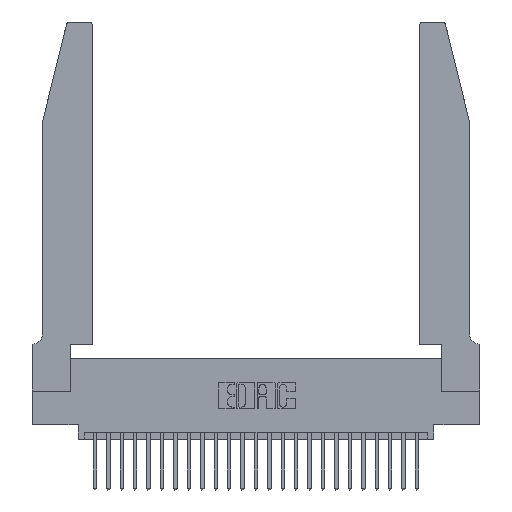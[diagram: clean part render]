
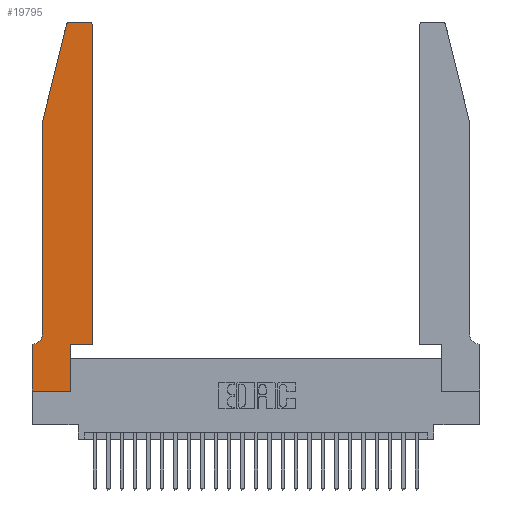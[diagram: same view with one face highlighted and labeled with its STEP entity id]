
A CAD part, top view. The second image highlights one B-rep face of the part: STEP entity #19795.
In plain terms, the highlighted planar face has unit normal (0, 0, 1).
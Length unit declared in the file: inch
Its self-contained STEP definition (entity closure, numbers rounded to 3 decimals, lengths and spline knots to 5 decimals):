
#88 = ORIENTED_EDGE ( 'NONE', *, *, #620, .T. ) ;
#238 = DIRECTION ( 'NONE',  ( 1., 0., 0. ) ) ;
#620 = EDGE_CURVE ( 'NONE', #8522, #22157, #18849, .T. ) ;
#905 = AXIS2_PLACEMENT_3D ( 'NONE', #3221, #17809, #5351 ) ;
#1166 = VECTOR ( 'NONE', #2863, 39.37008 ) ;
#1327 = VERTEX_POINT ( 'NONE', #24471 ) ;
#1481 = EDGE_CURVE ( 'NONE', #4591, #10371, #6172, .T. ) ;
#1505 = DIRECTION ( 'NONE',  ( 0., 1., 0. ) ) ;
#1758 = CARTESIAN_POINT ( 'NONE',  ( 0.0755, 0.35, 0.37 ) ) ;
#1765 = CARTESIAN_POINT ( 'NONE',  ( 0.2865, 0., 0.37 ) ) ;
#1898 = VECTOR ( 'NONE', #26459, 39.37008 ) ;
#2162 = ORIENTED_EDGE ( 'NONE', *, *, #11137, .T. ) ;
#2335 = VERTEX_POINT ( 'NONE', #6786 ) ;
#2593 = PLANE ( 'NONE',  #16353 ) ;
#2817 = LINE ( 'NONE', #15423, #1166 ) ;
#2863 = DIRECTION ( 'NONE',  ( 0., 1., 0. ) ) ;
#3044 = EDGE_CURVE ( 'NONE', #8219, #8522, #7078, .T. ) ;
#3221 = CARTESIAN_POINT ( 'NONE',  ( 0.4205, 2.72, 0.37 ) ) ;
#3338 = DIRECTION ( 'NONE',  ( 0., -1., 0. ) ) ;
#3476 = DIRECTION ( 'NONE',  ( 0., 0., -1. ) ) ;
#3484 = VECTOR ( 'NONE', #13917, 39.37008 ) ;
#4347 = ORIENTED_EDGE ( 'NONE', *, *, #3044, .T. ) ;
#4591 = VERTEX_POINT ( 'NONE', #17254 ) ;
#5323 = VECTOR ( 'NONE', #1505, 39.37008 ) ;
#5351 = DIRECTION ( 'NONE',  ( 1., 0., 0. ) ) ;
#6013 = LINE ( 'NONE', #14112, #5323 ) ;
#6172 = LINE ( 'NONE', #14824, #10483 ) ;
#6718 = CARTESIAN_POINT ( 'NONE',  ( 0.284, 2.72, 0.37 ) ) ;
#6786 = CARTESIAN_POINT ( 'NONE',  ( 0.4505, 2.72, 0.37 ) ) ;
#7078 = LINE ( 'NONE', #23524, #12006 ) ;
#7126 = ORIENTED_EDGE ( 'NONE', *, *, #12408, .T. ) ;
#7557 = ORIENTED_EDGE ( 'NONE', *, *, #21076, .T. ) ;
#7622 = CARTESIAN_POINT ( 'NONE',  ( 0.0755, 2., 0.37 ) ) ;
#7649 = VERTEX_POINT ( 'NONE', #11051 ) ;
#7797 = ORIENTED_EDGE ( 'NONE', *, *, #8776, .T. ) ;
#7857 = AXIS2_PLACEMENT_3D ( 'NONE', #16007, #3476, #18056 ) ;
#8028 = VERTEX_POINT ( 'NONE', #1765 ) ;
#8164 = CARTESIAN_POINT ( 'NONE',  ( 0.0755, 0.42, 0.37 ) ) ;
#8219 = VERTEX_POINT ( 'NONE', #20945 ) ;
#8522 = VERTEX_POINT ( 'NONE', #26108 ) ;
#8627 = DIRECTION ( 'NONE',  ( -0.239, -0.971, 0. ) ) ;
#8776 = EDGE_CURVE ( 'NONE', #22157, #7649, #20928, .T. ) ;
#9024 = DIRECTION ( 'NONE',  ( 0., 0., 1. ) ) ;
#9186 = AXIS2_PLACEMENT_3D ( 'NONE', #6718, #10730, #18779 ) ;
#9209 = CARTESIAN_POINT ( 'NONE',  ( 0.4505, 0.35, 0.37 ) ) ;
#9313 = CARTESIAN_POINT ( 'NONE',  ( 0., 0., 0.37 ) ) ;
#9957 = EDGE_CURVE ( 'NONE', #24139, #2335, #6013, .T. ) ;
#10061 = ORIENTED_EDGE ( 'NONE', *, *, #12568, .T. ) ;
#10371 = VERTEX_POINT ( 'NONE', #9313 ) ;
#10483 = VECTOR ( 'NONE', #12788, 39.37008 ) ;
#10730 = DIRECTION ( 'NONE',  ( 0., 0., 1. ) ) ;
#11051 = CARTESIAN_POINT ( 'NONE',  ( 0.0755, 2., 0.37 ) ) ;
#11137 = EDGE_CURVE ( 'NONE', #2335, #8219, #22070, .T. ) ;
#12006 = VECTOR ( 'NONE', #17447, 39.37008 ) ;
#12168 = VECTOR ( 'NONE', #3338, 39.37008 ) ;
#12408 = EDGE_CURVE ( 'NONE', #7649, #18172, #16973, .T. ) ;
#12568 = EDGE_CURVE ( 'NONE', #1327, #4591, #18542, .T. ) ;
#12788 = DIRECTION ( 'NONE',  ( 0., -1., 0. ) ) ;
#13130 = ORIENTED_EDGE ( 'NONE', *, *, #20721, .T. ) ;
#13458 = EDGE_LOOP ( 'NONE', ( #4347, #88, #7797, #7126, #13130, #10061, #26248, #21371, #19789, #7557, #18104, #2162 ) ) ;
#13691 = EDGE_CURVE ( 'NONE', #8028, #17243, #2817, .T. ) ;
#13917 = DIRECTION ( 'NONE',  ( 1., 0., 0. ) ) ;
#14112 = CARTESIAN_POINT ( 'NONE',  ( 0.4505, 0.35, 0.37 ) ) ;
#14824 = CARTESIAN_POINT ( 'NONE',  ( 0., 0., 0.37 ) ) ;
#15000 = CARTESIAN_POINT ( 'NONE',  ( 0.4505, 0.35, 0.37 ) ) ;
#15423 = CARTESIAN_POINT ( 'NONE',  ( 0.2865, 0.35, 0.37 ) ) ;
#16007 = CARTESIAN_POINT ( 'NONE',  ( 0.0055, 0.42, 0.37 ) ) ;
#16353 = AXIS2_PLACEMENT_3D ( 'NONE', #21298, #9024, #23300 ) ;
#16973 = LINE ( 'NONE', #7622, #12168 ) ;
#17243 = VERTEX_POINT ( 'NONE', #19490 ) ;
#17254 = CARTESIAN_POINT ( 'NONE',  ( 0., 0.35, 0.37 ) ) ;
#17447 = DIRECTION ( 'NONE',  ( -1., 0., 0. ) ) ;
#17542 = VECTOR ( 'NONE', #238, 39.37008 ) ;
#17809 = DIRECTION ( 'NONE',  ( 0., 0., 1. ) ) ;
#18056 = DIRECTION ( 'NONE',  ( -1., 0., 0. ) ) ;
#18104 = ORIENTED_EDGE ( 'NONE', *, *, #9957, .T. ) ;
#18172 = VERTEX_POINT ( 'NONE', #8164 ) ;
#18542 = LINE ( 'NONE', #1758, #1898 ) ;
#18779 = DIRECTION ( 'NONE',  ( 1., 0., 0. ) ) ;
#18849 = CIRCLE ( 'NONE', #9186, 0.03 ) ;
#19490 = CARTESIAN_POINT ( 'NONE',  ( 0.2865, 0.35, 0.37 ) ) ;
#19789 = ORIENTED_EDGE ( 'NONE', *, *, #13691, .T. ) ;
#19795 = ADVANCED_FACE ( 'NONE', ( #24963 ), #2593, .T. ) ;
#19978 = CARTESIAN_POINT ( 'NONE',  ( 0., 0., 0.37 ) ) ;
#20721 = EDGE_CURVE ( 'NONE', #18172, #1327, #24481, .T. ) ;
#20920 = CARTESIAN_POINT ( 'NONE',  ( 0.0755, 2., 0.37 ) ) ;
#20928 = LINE ( 'NONE', #20920, #26254 ) ;
#20945 = CARTESIAN_POINT ( 'NONE',  ( 0.4205, 2.75, 0.37 ) ) ;
#21030 = LINE ( 'NONE', #15000, #17542 ) ;
#21076 = EDGE_CURVE ( 'NONE', #17243, #24139, #21030, .T. ) ;
#21298 = CARTESIAN_POINT ( 'NONE',  ( 0., 0.35, 0.37 ) ) ;
#21359 = EDGE_CURVE ( 'NONE', #10371, #8028, #25403, .T. ) ;
#21371 = ORIENTED_EDGE ( 'NONE', *, *, #21359, .T. ) ;
#22070 = CIRCLE ( 'NONE', #905, 0.03 ) ;
#22157 = VERTEX_POINT ( 'NONE', #22955 ) ;
#22955 = CARTESIAN_POINT ( 'NONE',  ( 0.25487, 2.72718, 0.37 ) ) ;
#23300 = DIRECTION ( 'NONE',  ( 1., 0., 0. ) ) ;
#23524 = CARTESIAN_POINT ( 'NONE',  ( 0.2605, 2.75, 0.37 ) ) ;
#24139 = VERTEX_POINT ( 'NONE', #9209 ) ;
#24471 = CARTESIAN_POINT ( 'NONE',  ( 0.0055, 0.35, 0.37 ) ) ;
#24481 = CIRCLE ( 'NONE', #7857, 0.07 ) ;
#24963 = FACE_OUTER_BOUND ( 'NONE', #13458, .T. ) ;
#25403 = LINE ( 'NONE', #19978, #3484 ) ;
#26108 = CARTESIAN_POINT ( 'NONE',  ( 0.284, 2.75, 0.37 ) ) ;
#26248 = ORIENTED_EDGE ( 'NONE', *, *, #1481, .T. ) ;
#26254 = VECTOR ( 'NONE', #8627, 39.37008 ) ;
#26459 = DIRECTION ( 'NONE',  ( -1., 0., 0. ) ) ;
